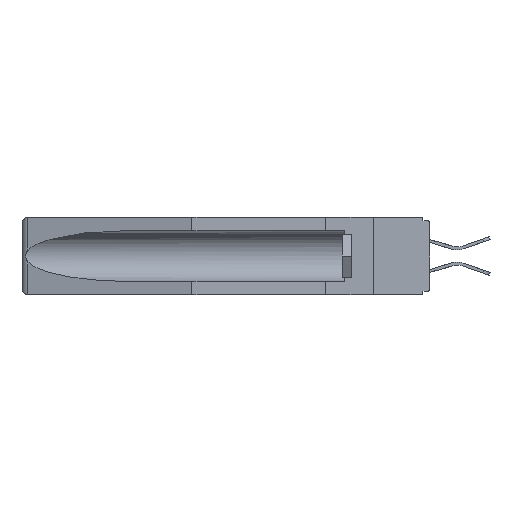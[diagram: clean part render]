
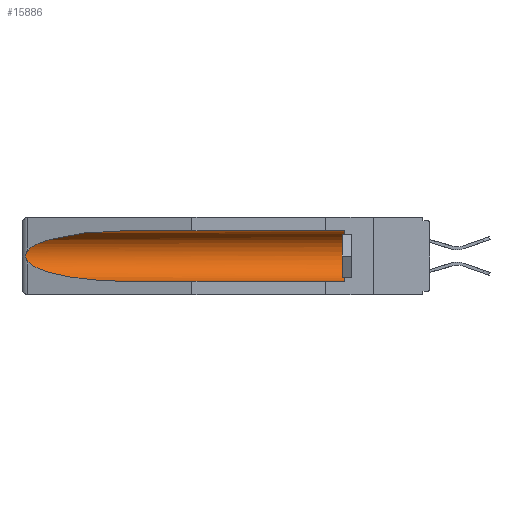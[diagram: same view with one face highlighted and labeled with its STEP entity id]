
A CAD part, left-side view. The second image highlights one B-rep face of the part: STEP entity #15886.
In plain terms, the highlighted cylindrical face has radius 2.857 mm (diameter 5.715 mm), a partial arc.
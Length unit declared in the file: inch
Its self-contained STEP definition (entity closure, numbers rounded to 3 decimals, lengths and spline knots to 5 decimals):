
#320 = CARTESIAN_POINT ( 'NONE',  ( 0.155, -0.30754, -0.1715 ) ) ;
#413 = AXIS2_PLACEMENT_3D ( 'NONE', #320, #10487, #2269 ) ;
#830 = CARTESIAN_POINT ( 'NONE',  ( 0.2675, 1.53308, -0.16763 ) ) ;
#2269 = DIRECTION ( 'NONE',  ( 0., 0., 1. ) ) ;
#2412 = CARTESIAN_POINT ( 'NONE',  ( 0.26537, 1.52718, -0.19328 ) ) ;
#2703 = CARTESIAN_POINT ( 'NONE',  ( 0.2675, 1.53308, -0.17534 ) ) ;
#2772 = EDGE_CURVE ( 'NONE', #13023, #11311, #17464, .T. ) ;
#3050 = CARTESIAN_POINT ( 'NONE',  ( 0.26537, 1.52718, -0.14972 ) ) ;
#4545 = EDGE_CURVE ( 'NONE', #25377, #10131, #17343, .T. ) ;
#4779 = CARTESIAN_POINT ( 'NONE',  ( 0.155, 1.07973, -0.284 ) ) ;
#5126 = ORIENTED_EDGE ( 'NONE', *, *, #2772, .T. ) ;
#5285 = DIRECTION ( 'NONE',  ( 0., 1., 0. ) ) ;
#5410 = ORIENTED_EDGE ( 'NONE', *, *, #4545, .F. ) ;
#6840 = ORIENTED_EDGE ( 'NONE', *, *, #14931, .T. ) ;
#7063 = CARTESIAN_POINT ( 'NONE',  ( 0.26597, 1.52961, -0.15275 ) ) ;
#7698 = CYLINDRICAL_SURFACE ( 'NONE', #413, 0.1125 ) ;
#8759 = CARTESIAN_POINT ( 'NONE',  ( 0.155, 1.07973, -0.284 ) ) ;
#8967 = EDGE_CURVE ( 'NONE', #18630, #19163, #17809, .T. ) ;
#9116 = CARTESIAN_POINT ( 'NONE',  ( 0.25451, 1.48313, -0.09465 ) ) ;
#9498 = DIRECTION ( 'NONE',  ( 0., 1., 0. ) ) ;
#9896 = AXIS2_PLACEMENT_3D ( 'NONE', #17118, #11057, #17204 ) ;
#10131 = VERTEX_POINT ( 'NONE', #4779 ) ;
#10487 = DIRECTION ( 'NONE',  ( 0., 1., 0. ) ) ;
#11057 = DIRECTION ( 'NONE',  ( 0., -1., 0. ) ) ;
#11311 = VERTEX_POINT ( 'NONE', #2412 ) ;
#11398 = EDGE_CURVE ( 'NONE', #11311, #10131, #12721, .T. ) ;
#11472 = EDGE_CURVE ( 'NONE', #25377, #18630, #12576, .T. ) ;
#12576 = CIRCLE ( 'NONE', #9896, 0.1125 ) ;
#12721 =( BOUNDED_CURVE ( )  B_SPLINE_CURVE ( 3, ( #22671, #24937, #20860, #8759 ),
 .UNSPECIFIED., .F., .T. ) 
 B_SPLINE_CURVE_WITH_KNOTS ( ( 4, 4 ),
 ( 0.1948, 1.5708 ),
 .UNSPECIFIED. ) 
 CURVE ( )  GEOMETRIC_REPRESENTATION_ITEM ( )  RATIONAL_B_SPLINE_CURVE ( ( 1., 0.848, 0.848, 1. ) ) 
 REPRESENTATION_ITEM ( '' )  );
#13023 = VERTEX_POINT ( 'NONE', #22224 ) ;
#13116 = FACE_OUTER_BOUND ( 'NONE', #13900, .T. ) ;
#13197 = VECTOR ( 'NONE', #9498, 39.37008 ) ;
#13205 = CARTESIAN_POINT ( 'NONE',  ( 0.26654, 1.53092, -0.15636 ) ) ;
#13900 = EDGE_LOOP ( 'NONE', ( #6840, #5126, #20868, #5410, #20100, #17162 ) ) ;
#14931 = EDGE_CURVE ( 'NONE', #19163, #13023, #20239, .T. ) ;
#15162 = CARTESIAN_POINT ( 'NONE',  ( 0.155, 1.07973, -0.059 ) ) ;
#15886 = ADVANCED_FACE ( 'NONE', ( #13116 ), #7698, .F. ) ;
#16312 = CARTESIAN_POINT ( 'NONE',  ( 0.155, 1.07973, -0.059 ) ) ;
#16967 = CARTESIAN_POINT ( 'NONE',  ( 0.26655, 1.53094, -0.18657 ) ) ;
#17046 = CARTESIAN_POINT ( 'NONE',  ( 0.21114, 1.30732, -0.059 ) ) ;
#17118 = CARTESIAN_POINT ( 'NONE',  ( 0.155, 0.126, -0.1715 ) ) ;
#17144 = CARTESIAN_POINT ( 'NONE',  ( 0.26597, 1.5296, -0.19026 ) ) ;
#17162 = ORIENTED_EDGE ( 'NONE', *, *, #8967, .T. ) ;
#17189 = CARTESIAN_POINT ( 'NONE',  ( 0.155, 0.126, -0.284 ) ) ;
#17204 = DIRECTION ( 'NONE',  ( 0., 0., 1. ) ) ;
#17343 = LINE ( 'NONE', #19646, #13197 ) ;
#17464 = B_SPLINE_CURVE_WITH_KNOTS ( 'NONE', 3,
 ( #23316, #7063, #13205, #23139, #830, #2703, #18947, #16967, #17144, #23230 ),
 .UNSPECIFIED., .F., .F.,
 ( 4, 2, 2, 2, 4 ),
 ( 0., 0.00029, 0.00058, 0.00087, 0.00117 ),
 .UNSPECIFIED. ) ;
#17809 = LINE ( 'NONE', #21852, #18791 ) ;
#18630 = VERTEX_POINT ( 'NONE', #25064 ) ;
#18791 = VECTOR ( 'NONE', #5285, 39.37008 ) ;
#18947 = CARTESIAN_POINT ( 'NONE',  ( 0.2673, 1.53269, -0.17917 ) ) ;
#19163 = VERTEX_POINT ( 'NONE', #16312 ) ;
#19646 = CARTESIAN_POINT ( 'NONE',  ( 0.155, -0.30754, -0.284 ) ) ;
#20100 = ORIENTED_EDGE ( 'NONE', *, *, #11472, .T. ) ;
#20239 =( BOUNDED_CURVE ( )  B_SPLINE_CURVE ( 3, ( #15162, #17046, #9116, #3050 ),
 .UNSPECIFIED., .F., .F. ) 
 B_SPLINE_CURVE_WITH_KNOTS ( ( 4, 4 ),
 ( 4.71239, 6.08839 ),
 .UNSPECIFIED. ) 
 CURVE ( )  GEOMETRIC_REPRESENTATION_ITEM ( )  RATIONAL_B_SPLINE_CURVE ( ( 1., 0.848, 0.848, 1. ) ) 
 REPRESENTATION_ITEM ( '' )  );
#20860 = CARTESIAN_POINT ( 'NONE',  ( 0.21114, 1.30732, -0.284 ) ) ;
#20868 = ORIENTED_EDGE ( 'NONE', *, *, #11398, .T. ) ;
#21852 = CARTESIAN_POINT ( 'NONE',  ( 0.155, -0.30754, -0.059 ) ) ;
#22224 = CARTESIAN_POINT ( 'NONE',  ( 0.26537, 1.52718, -0.14972 ) ) ;
#22671 = CARTESIAN_POINT ( 'NONE',  ( 0.26537, 1.52718, -0.19328 ) ) ;
#23139 = CARTESIAN_POINT ( 'NONE',  ( 0.2673, 1.5327, -0.16383 ) ) ;
#23230 = CARTESIAN_POINT ( 'NONE',  ( 0.26537, 1.52718, -0.19328 ) ) ;
#23316 = CARTESIAN_POINT ( 'NONE',  ( 0.26537, 1.52718, -0.14972 ) ) ;
#24937 = CARTESIAN_POINT ( 'NONE',  ( 0.25451, 1.48313, -0.24835 ) ) ;
#25064 = CARTESIAN_POINT ( 'NONE',  ( 0.155, 0.126, -0.059 ) ) ;
#25377 = VERTEX_POINT ( 'NONE', #17189 ) ;
